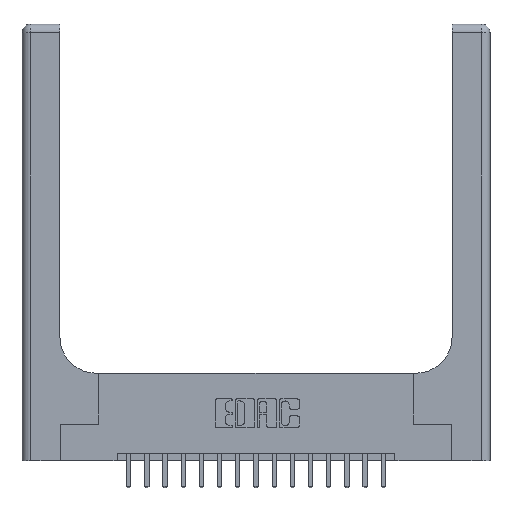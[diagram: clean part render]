
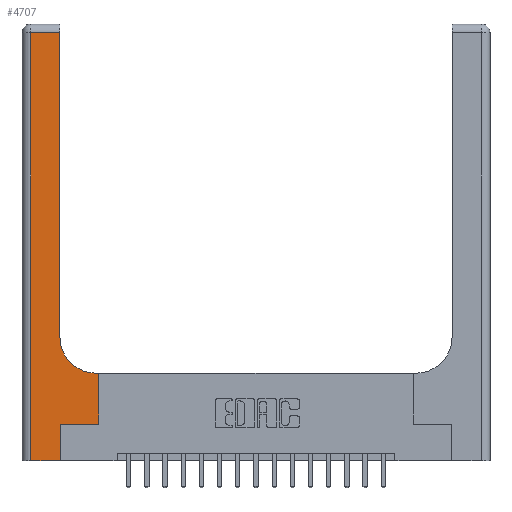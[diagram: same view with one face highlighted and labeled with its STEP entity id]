
A CAD part, top view. The second image highlights one B-rep face of the part: STEP entity #4707.
In plain terms, the highlighted planar face has unit normal (0, 0, 1).
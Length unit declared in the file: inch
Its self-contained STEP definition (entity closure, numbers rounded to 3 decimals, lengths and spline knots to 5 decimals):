
#470 = DIRECTION ( 'NONE',  ( 0., 0., -1. ) ) ;
#726 = EDGE_CURVE ( 'NONE', #18908, #1098, #3502, .T. ) ;
#1098 = VERTEX_POINT ( 'NONE', #6392 ) ;
#1184 = CIRCLE ( 'NONE', #1809, 0.25 ) ;
#1209 = DIRECTION ( 'NONE',  ( -1., 0., 0. ) ) ;
#1503 = EDGE_CURVE ( 'NONE', #17998, #1924, #6081, .T. ) ;
#1809 = AXIS2_PLACEMENT_3D ( 'NONE', #13461, #470, #15213 ) ;
#1916 = DIRECTION ( 'NONE',  ( 0., 1., 0. ) ) ;
#1924 = VERTEX_POINT ( 'NONE', #18348 ) ;
#2651 = VECTOR ( 'NONE', #13077, 39.37008 ) ;
#2662 = CARTESIAN_POINT ( 'NONE',  ( 0.26, 0.6, 0.37 ) ) ;
#2816 = CARTESIAN_POINT ( 'NONE',  ( 0.265, 0.25, 0.37 ) ) ;
#3117 = DIRECTION ( 'NONE',  ( 0., 1., 0. ) ) ;
#3502 = LINE ( 'NONE', #12235, #14107 ) ;
#3697 = DIRECTION ( 'NONE',  ( -1., 0., 0. ) ) ;
#4707 = ADVANCED_FACE ( 'NONE', ( #9821 ), #18722, .F. ) ;
#4714 = CARTESIAN_POINT ( 'NONE',  ( 0.265, 0., 0.37 ) ) ;
#5322 = ORIENTED_EDGE ( 'NONE', *, *, #14915, .T. ) ;
#5495 = CARTESIAN_POINT ( 'NONE',  ( 0.51, 0.6, 0.37 ) ) ;
#5555 = EDGE_LOOP ( 'NONE', ( #8450, #17592, #12952, #11820, #18816, #5322, #8283, #7760, #11300 ) ) ;
#5910 = DIRECTION ( 'NONE',  ( -1., 0., 0. ) ) ;
#6081 = LINE ( 'NONE', #4714, #6738 ) ;
#6392 = CARTESIAN_POINT ( 'NONE',  ( 0.26, 2.94, 0.37 ) ) ;
#6738 = VECTOR ( 'NONE', #1916, 39.37008 ) ;
#6817 = DIRECTION ( 'NONE',  ( 1., 0., 0. ) ) ;
#7196 = EDGE_CURVE ( 'NONE', #18414, #11134, #8631, .T. ) ;
#7380 = DIRECTION ( 'NONE',  ( 0., 0., -1. ) ) ;
#7760 = ORIENTED_EDGE ( 'NONE', *, *, #10196, .T. ) ;
#8070 = LINE ( 'NONE', #12515, #16641 ) ;
#8172 = DIRECTION ( 'NONE',  ( 0., 1., 0. ) ) ;
#8283 = ORIENTED_EDGE ( 'NONE', *, *, #18268, .T. ) ;
#8450 = ORIENTED_EDGE ( 'NONE', *, *, #726, .T. ) ;
#8631 = LINE ( 'NONE', #14536, #2651 ) ;
#8958 = VECTOR ( 'NONE', #6817, 39.37008 ) ;
#9252 = CARTESIAN_POINT ( 'NONE',  ( 0.265, 0., 0.37 ) ) ;
#9821 = FACE_OUTER_BOUND ( 'NONE', #5555, .T. ) ;
#10196 = EDGE_CURVE ( 'NONE', #12954, #19074, #17384, .T. ) ;
#11123 = CARTESIAN_POINT ( 'NONE',  ( 0.26, 0.85, 0.37 ) ) ;
#11134 = VERTEX_POINT ( 'NONE', #15188 ) ;
#11300 = ORIENTED_EDGE ( 'NONE', *, *, #12365, .T. ) ;
#11550 = LINE ( 'NONE', #19003, #14532 ) ;
#11727 = DIRECTION ( 'NONE',  ( 1., 0., 0. ) ) ;
#11820 = ORIENTED_EDGE ( 'NONE', *, *, #13604, .T. ) ;
#12165 = EDGE_CURVE ( 'NONE', #1098, #18414, #8070, .T. ) ;
#12235 = CARTESIAN_POINT ( 'NONE',  ( 0.26, 3., 0.37 ) ) ;
#12238 = CARTESIAN_POINT ( 'NONE',  ( 0.528, 0.25, 0.37 ) ) ;
#12365 = EDGE_CURVE ( 'NONE', #19074, #18908, #1184, .T. ) ;
#12515 = CARTESIAN_POINT ( 'NONE',  ( 0., 2.94, 0.37 ) ) ;
#12952 = ORIENTED_EDGE ( 'NONE', *, *, #7196, .T. ) ;
#12954 = VERTEX_POINT ( 'NONE', #14198 ) ;
#13077 = DIRECTION ( 'NONE',  ( 0., -1., 0. ) ) ;
#13367 = VERTEX_POINT ( 'NONE', #12238 ) ;
#13380 = CARTESIAN_POINT ( 'NONE',  ( 0.06, 2.94, 0.37 ) ) ;
#13461 = CARTESIAN_POINT ( 'NONE',  ( 0.51, 0.85, 0.37 ) ) ;
#13604 = EDGE_CURVE ( 'NONE', #11134, #17998, #11550, .T. ) ;
#13853 = AXIS2_PLACEMENT_3D ( 'NONE', #14838, #7380, #5910 ) ;
#13988 = CARTESIAN_POINT ( 'NONE',  ( 0.528, 0.25, 0.37 ) ) ;
#14107 = VECTOR ( 'NONE', #3117, 39.37008 ) ;
#14198 = CARTESIAN_POINT ( 'NONE',  ( 0.528, 0.6, 0.37 ) ) ;
#14532 = VECTOR ( 'NONE', #11727, 39.37008 ) ;
#14536 = CARTESIAN_POINT ( 'NONE',  ( 0.06, 3., 0.37 ) ) ;
#14838 = CARTESIAN_POINT ( 'NONE',  ( 0., 3., 0.37 ) ) ;
#14915 = EDGE_CURVE ( 'NONE', #1924, #13367, #17543, .T. ) ;
#15188 = CARTESIAN_POINT ( 'NONE',  ( 0.06, 0., 0.37 ) ) ;
#15213 = DIRECTION ( 'NONE',  ( 1., 0., 0. ) ) ;
#15626 = LINE ( 'NONE', #13988, #16756 ) ;
#16641 = VECTOR ( 'NONE', #3697, 39.37008 ) ;
#16756 = VECTOR ( 'NONE', #8172, 39.37008 ) ;
#17384 = LINE ( 'NONE', #2662, #18152 ) ;
#17543 = LINE ( 'NONE', #2816, #8958 ) ;
#17592 = ORIENTED_EDGE ( 'NONE', *, *, #12165, .T. ) ;
#17998 = VERTEX_POINT ( 'NONE', #9252 ) ;
#18152 = VECTOR ( 'NONE', #1209, 39.37008 ) ;
#18268 = EDGE_CURVE ( 'NONE', #13367, #12954, #15626, .T. ) ;
#18348 = CARTESIAN_POINT ( 'NONE',  ( 0.265, 0.25, 0.37 ) ) ;
#18414 = VERTEX_POINT ( 'NONE', #13380 ) ;
#18722 = PLANE ( 'NONE',  #13853 ) ;
#18816 = ORIENTED_EDGE ( 'NONE', *, *, #1503, .T. ) ;
#18908 = VERTEX_POINT ( 'NONE', #11123 ) ;
#19003 = CARTESIAN_POINT ( 'NONE',  ( 0., 0., 0.37 ) ) ;
#19074 = VERTEX_POINT ( 'NONE', #5495 ) ;
